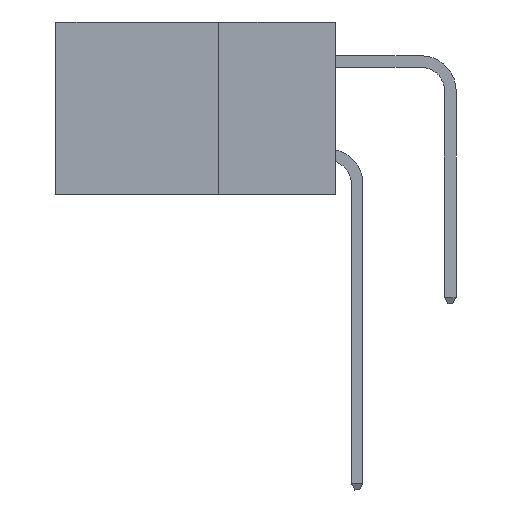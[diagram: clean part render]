
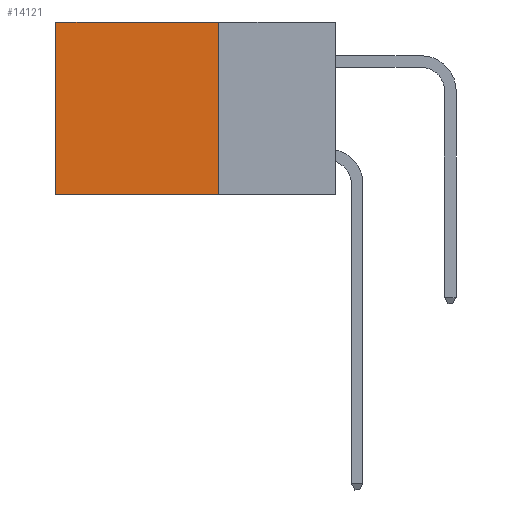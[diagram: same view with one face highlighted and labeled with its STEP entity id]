
A CAD part, left-side view. The second image highlights one B-rep face of the part: STEP entity #14121.
In plain terms, the highlighted planar face has unit normal (-1, 0, 0).
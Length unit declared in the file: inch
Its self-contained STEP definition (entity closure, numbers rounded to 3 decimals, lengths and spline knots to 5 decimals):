
#1057 = VERTEX_POINT ( 'NONE', #25115 ) ;
#1131 = EDGE_CURVE ( 'NONE', #20802, #16190, #6362, .T. ) ;
#1386 = AXIS2_PLACEMENT_3D ( 'NONE', #21389, #17416, #6705 ) ;
#2499 = VECTOR ( 'NONE', #12789, 39.37008 ) ;
#3125 = CARTESIAN_POINT ( 'NONE',  ( 0.2875, 0.25, 0. ) ) ;
#3502 = LINE ( 'NONE', #22369, #2499 ) ;
#3871 = VECTOR ( 'NONE', #25732, 39.37008 ) ;
#4035 = PLANE ( 'NONE',  #1386 ) ;
#4474 = CARTESIAN_POINT ( 'NONE',  ( 0.2875, 0.25, 0. ) ) ;
#4516 = ORIENTED_EDGE ( 'NONE', *, *, #9999, .F. ) ;
#5710 = VECTOR ( 'NONE', #23055, 39.37008 ) ;
#6362 = LINE ( 'NONE', #22971, #5710 ) ;
#6421 = EDGE_LOOP ( 'NONE', ( #24416, #11346, #4516, #24106 ) ) ;
#6705 = DIRECTION ( 'NONE',  ( 0., 0., -1. ) ) ;
#7542 = CARTESIAN_POINT ( 'NONE',  ( 0.2875, 0.6, -0.37 ) ) ;
#9999 = EDGE_CURVE ( 'NONE', #10616, #1057, #19256, .T. ) ;
#10616 = VERTEX_POINT ( 'NONE', #3125 ) ;
#11346 = ORIENTED_EDGE ( 'NONE', *, *, #19370, .F. ) ;
#11603 = CARTESIAN_POINT ( 'NONE',  ( 0.2875, 0.25, 0. ) ) ;
#12789 = DIRECTION ( 'NONE',  ( 0., 1., 0. ) ) ;
#14121 = ADVANCED_FACE ( 'NONE', ( #22594 ), #4035, .F. ) ;
#16190 = VERTEX_POINT ( 'NONE', #7542 ) ;
#17416 = DIRECTION ( 'NONE',  ( 1., 0., 0. ) ) ;
#18350 = DIRECTION ( 'NONE',  ( 0., 0., -1. ) ) ;
#19256 = LINE ( 'NONE', #4474, #24725 ) ;
#19370 = EDGE_CURVE ( 'NONE', #1057, #16190, #3502, .T. ) ;
#20802 = VERTEX_POINT ( 'NONE', #24548 ) ;
#21389 = CARTESIAN_POINT ( 'NONE',  ( 0.2875, 0.25, 0. ) ) ;
#22369 = CARTESIAN_POINT ( 'NONE',  ( 0.2875, 0.25, -0.37 ) ) ;
#22594 = FACE_OUTER_BOUND ( 'NONE', #6421, .T. ) ;
#22971 = CARTESIAN_POINT ( 'NONE',  ( 0.2875, 0.6, 0. ) ) ;
#23055 = DIRECTION ( 'NONE',  ( 0., 0., -1. ) ) ;
#24106 = ORIENTED_EDGE ( 'NONE', *, *, #25622, .T. ) ;
#24416 = ORIENTED_EDGE ( 'NONE', *, *, #1131, .T. ) ;
#24548 = CARTESIAN_POINT ( 'NONE',  ( 0.2875, 0.6, 0. ) ) ;
#24725 = VECTOR ( 'NONE', #18350, 39.37008 ) ;
#24869 = LINE ( 'NONE', #11603, #3871 ) ;
#25115 = CARTESIAN_POINT ( 'NONE',  ( 0.2875, 0.25, -0.37 ) ) ;
#25622 = EDGE_CURVE ( 'NONE', #10616, #20802, #24869, .T. ) ;
#25732 = DIRECTION ( 'NONE',  ( 0., 1., 0. ) ) ;
